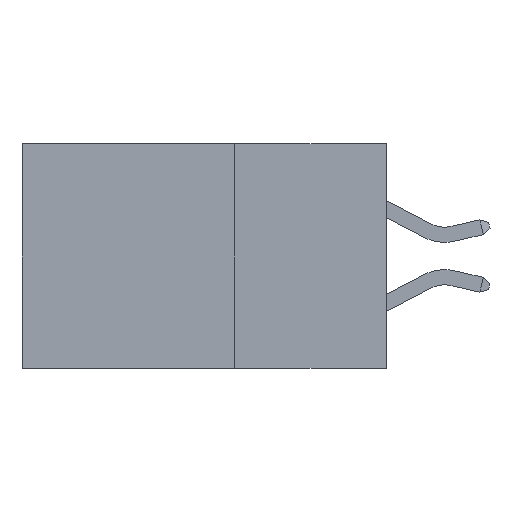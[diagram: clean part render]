
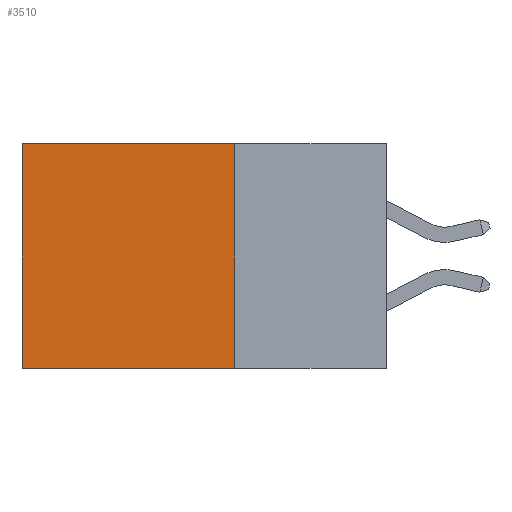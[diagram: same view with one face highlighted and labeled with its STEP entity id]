
A CAD part, left-side view. The second image highlights one B-rep face of the part: STEP entity #3510.
In plain terms, the highlighted planar face has unit normal (-1, 0, 0).
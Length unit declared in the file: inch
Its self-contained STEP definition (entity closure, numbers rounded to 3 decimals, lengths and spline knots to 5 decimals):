
#261 = DIRECTION ( 'NONE',  ( 0., 1., 0. ) ) ;
#474 = CARTESIAN_POINT ( 'NONE',  ( 0.2615, 0.6, -0.37 ) ) ;
#1199 = CARTESIAN_POINT ( 'NONE',  ( 0.2615, 0.25, -0.37 ) ) ;
#1339 = VERTEX_POINT ( 'NONE', #2158 ) ;
#1385 = EDGE_LOOP ( 'NONE', ( #3422, #3103, #7829, #2910 ) ) ;
#2158 = CARTESIAN_POINT ( 'NONE',  ( 0.2615, 0.25, -0.37 ) ) ;
#2383 = DIRECTION ( 'NONE',  ( 0., 0., -1. ) ) ;
#2649 = FACE_OUTER_BOUND ( 'NONE', #1385, .T. ) ;
#2718 = VECTOR ( 'NONE', #261, 39.37008 ) ;
#2910 = ORIENTED_EDGE ( 'NONE', *, *, #9984, .T. ) ;
#3103 = ORIENTED_EDGE ( 'NONE', *, *, #10694, .F. ) ;
#3130 = DIRECTION ( 'NONE',  ( 0., 0., -1. ) ) ;
#3235 = VECTOR ( 'NONE', #7964, 39.37008 ) ;
#3326 = EDGE_CURVE ( 'NONE', #6656, #1339, #4656, .T. ) ;
#3422 = ORIENTED_EDGE ( 'NONE', *, *, #6257, .T. ) ;
#3510 = ADVANCED_FACE ( 'NONE', ( #2649 ), #9075, .F. ) ;
#4656 = LINE ( 'NONE', #10956, #6792 ) ;
#4821 = LINE ( 'NONE', #7970, #3235 ) ;
#4903 = AXIS2_PLACEMENT_3D ( 'NONE', #1199, #11228, #2383 ) ;
#4921 = CARTESIAN_POINT ( 'NONE',  ( 0.2615, 0.25, -0.37 ) ) ;
#6067 = CARTESIAN_POINT ( 'NONE',  ( 0.2615, 0.25, 0. ) ) ;
#6257 = EDGE_CURVE ( 'NONE', #10839, #7861, #4821, .T. ) ;
#6656 = VERTEX_POINT ( 'NONE', #6067 ) ;
#6792 = VECTOR ( 'NONE', #3130, 39.37008 ) ;
#6954 = CARTESIAN_POINT ( 'NONE',  ( 0.2615, 0.6, 0. ) ) ;
#7829 = ORIENTED_EDGE ( 'NONE', *, *, #3326, .F. ) ;
#7861 = VERTEX_POINT ( 'NONE', #474 ) ;
#7964 = DIRECTION ( 'NONE',  ( 0., 0., -1. ) ) ;
#7970 = CARTESIAN_POINT ( 'NONE',  ( 0.2615, 0.6, -0.37 ) ) ;
#8490 = CARTESIAN_POINT ( 'NONE',  ( 0.2615, 0.25, 0. ) ) ;
#9075 = PLANE ( 'NONE',  #4903 ) ;
#9407 = DIRECTION ( 'NONE',  ( 0., 1., 0. ) ) ;
#9984 = EDGE_CURVE ( 'NONE', #6656, #10839, #11523, .T. ) ;
#10044 = LINE ( 'NONE', #4921, #2718 ) ;
#10694 = EDGE_CURVE ( 'NONE', #1339, #7861, #10044, .T. ) ;
#10839 = VERTEX_POINT ( 'NONE', #6954 ) ;
#10956 = CARTESIAN_POINT ( 'NONE',  ( 0.2615, 0.25, -0.37 ) ) ;
#11228 = DIRECTION ( 'NONE',  ( 1., 0., 0. ) ) ;
#11241 = VECTOR ( 'NONE', #9407, 39.37008 ) ;
#11523 = LINE ( 'NONE', #8490, #11241 ) ;
